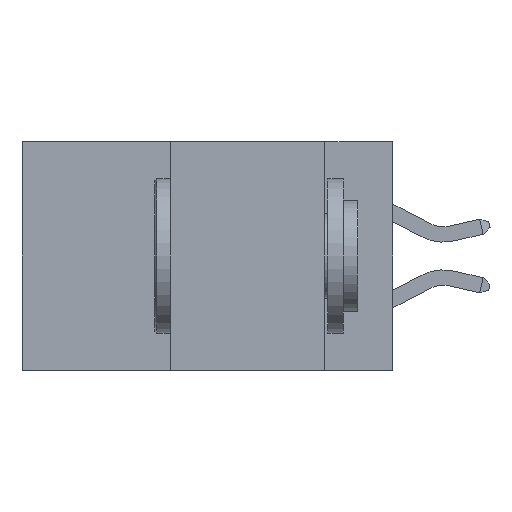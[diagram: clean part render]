
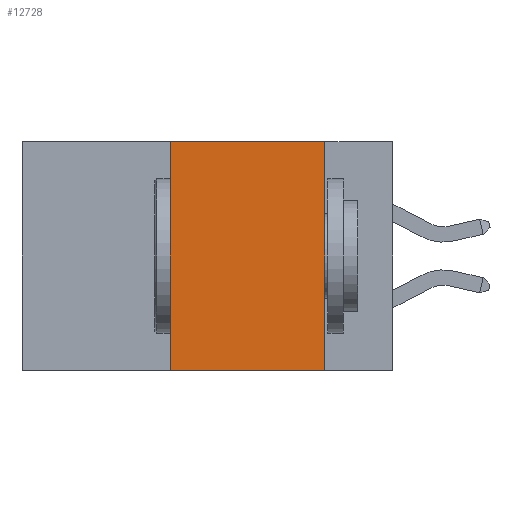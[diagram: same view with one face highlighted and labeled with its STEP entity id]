
A CAD part, left-side view. The second image highlights one B-rep face of the part: STEP entity #12728.
In plain terms, the highlighted planar face has unit normal (-1, 0, 0).
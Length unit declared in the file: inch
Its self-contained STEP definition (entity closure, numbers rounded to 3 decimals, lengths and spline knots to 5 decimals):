
#1321 = ORIENTED_EDGE ( 'NONE', *, *, #4536, .F. ) ;
#1335 = EDGE_LOOP ( 'NONE', ( #12403, #7415, #1321, #16191 ) ) ;
#1373 = DIRECTION ( 'NONE',  ( 0., 0., -1. ) ) ;
#2640 = CARTESIAN_POINT ( 'NONE',  ( 0., 0.6, -0.37 ) ) ;
#3666 = CARTESIAN_POINT ( 'NONE',  ( 0., 0.11, 0. ) ) ;
#3694 = VECTOR ( 'NONE', #12129, 39.37008 ) ;
#4536 = EDGE_CURVE ( 'NONE', #8743, #9344, #18005, .T. ) ;
#4653 = CARTESIAN_POINT ( 'NONE',  ( 0., 0.6, 0. ) ) ;
#4663 = AXIS2_PLACEMENT_3D ( 'NONE', #9212, #11970, #1373 ) ;
#5448 = DIRECTION ( 'NONE',  ( 0., 0., -1. ) ) ;
#6224 = CARTESIAN_POINT ( 'NONE',  ( 0., 0.36, 0. ) ) ;
#7415 = ORIENTED_EDGE ( 'NONE', *, *, #14387, .F. ) ;
#8743 = VERTEX_POINT ( 'NONE', #14427 ) ;
#9156 = LINE ( 'NONE', #3666, #12612 ) ;
#9212 = CARTESIAN_POINT ( 'NONE',  ( 0., 0.6, 0. ) ) ;
#9344 = VERTEX_POINT ( 'NONE', #6224 ) ;
#10313 = EDGE_CURVE ( 'NONE', #12513, #12377, #9156, .T. ) ;
#11375 = VECTOR ( 'NONE', #19500, 39.37008 ) ;
#11923 = LINE ( 'NONE', #4653, #18025 ) ;
#11970 = DIRECTION ( 'NONE',  ( 1., 0., 0. ) ) ;
#12129 = DIRECTION ( 'NONE',  ( 0., -1., 0. ) ) ;
#12377 = VERTEX_POINT ( 'NONE', #17522 ) ;
#12403 = ORIENTED_EDGE ( 'NONE', *, *, #10313, .F. ) ;
#12513 = VERTEX_POINT ( 'NONE', #13274 ) ;
#12559 = LINE ( 'NONE', #2640, #3694 ) ;
#12612 = VECTOR ( 'NONE', #5448, 39.37008 ) ;
#12728 = ADVANCED_FACE ( 'NONE', ( #18898 ), #18264, .F. ) ;
#13274 = CARTESIAN_POINT ( 'NONE',  ( 0., 0.11, 0. ) ) ;
#14387 = EDGE_CURVE ( 'NONE', #9344, #12513, #11923, .T. ) ;
#14427 = CARTESIAN_POINT ( 'NONE',  ( 0., 0.36, -0.37 ) ) ;
#16191 = ORIENTED_EDGE ( 'NONE', *, *, #17490, .T. ) ;
#17490 = EDGE_CURVE ( 'NONE', #8743, #12377, #12559, .T. ) ;
#17522 = CARTESIAN_POINT ( 'NONE',  ( 0., 0.11, -0.37 ) ) ;
#17728 = CARTESIAN_POINT ( 'NONE',  ( 0., 0.36, 0. ) ) ;
#18005 = LINE ( 'NONE', #17728, #11375 ) ;
#18025 = VECTOR ( 'NONE', #20328, 39.37008 ) ;
#18264 = PLANE ( 'NONE',  #4663 ) ;
#18898 = FACE_OUTER_BOUND ( 'NONE', #1335, .T. ) ;
#19500 = DIRECTION ( 'NONE',  ( 0., 0., 1. ) ) ;
#20328 = DIRECTION ( 'NONE',  ( 0., -1., 0. ) ) ;
